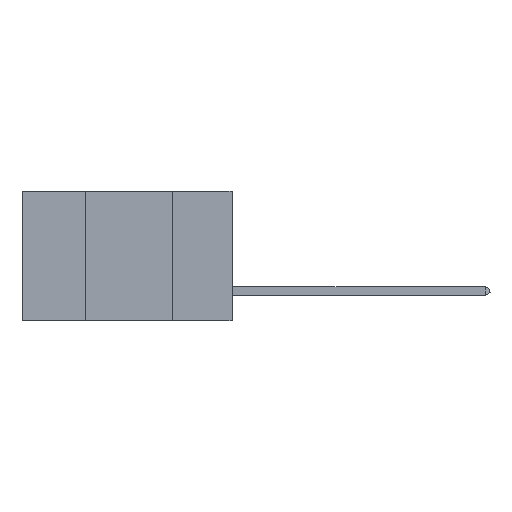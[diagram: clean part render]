
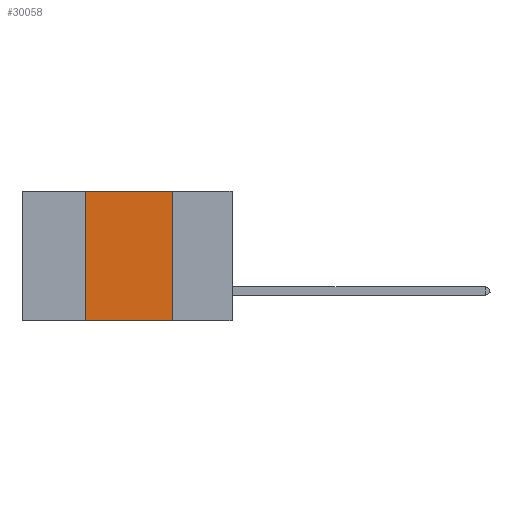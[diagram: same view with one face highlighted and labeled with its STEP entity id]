
A CAD part, left-side view. The second image highlights one B-rep face of the part: STEP entity #30058.
In plain terms, the highlighted planar face has unit normal (-1, 0, 0).
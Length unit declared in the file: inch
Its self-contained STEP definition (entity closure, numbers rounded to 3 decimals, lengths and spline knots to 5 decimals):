
#289 = VERTEX_POINT ( 'NONE', #24960 ) ;
#2509 = DIRECTION ( 'NONE',  ( 0., 0., 1. ) ) ;
#3548 = DIRECTION ( 'NONE',  ( 1., 0., 0. ) ) ;
#4126 = CARTESIAN_POINT ( 'NONE',  ( 0., 0.42, 0. ) ) ;
#5103 = ORIENTED_EDGE ( 'NONE', *, *, #31413, .F. ) ;
#5664 = LINE ( 'NONE', #14095, #44110 ) ;
#5711 = CARTESIAN_POINT ( 'NONE',  ( 0., 0.6, 0. ) ) ;
#10487 = VECTOR ( 'NONE', #16768, 39.37008 ) ;
#10623 = EDGE_LOOP ( 'NONE', ( #30626, #41800, #5103, #26706 ) ) ;
#14095 = CARTESIAN_POINT ( 'NONE',  ( 0., 0.42, 0. ) ) ;
#14500 = DIRECTION ( 'NONE',  ( 0., 0., -1. ) ) ;
#16768 = DIRECTION ( 'NONE',  ( 0., 0., -1. ) ) ;
#18489 = VERTEX_POINT ( 'NONE', #28493 ) ;
#20964 = EDGE_CURVE ( 'NONE', #289, #18489, #33792, .T. ) ;
#22131 = CARTESIAN_POINT ( 'NONE',  ( 0., 0.6, 0. ) ) ;
#24960 = CARTESIAN_POINT ( 'NONE',  ( 0., 0.17, 0. ) ) ;
#25874 = PLANE ( 'NONE',  #47348 ) ;
#26318 = CARTESIAN_POINT ( 'NONE',  ( 0., 0.6, -0.37 ) ) ;
#26706 = ORIENTED_EDGE ( 'NONE', *, *, #45067, .T. ) ;
#26965 = VECTOR ( 'NONE', #35706, 39.37008 ) ;
#28493 = CARTESIAN_POINT ( 'NONE',  ( 0., 0.17, -0.37 ) ) ;
#28886 = VERTEX_POINT ( 'NONE', #45642 ) ;
#29574 = DIRECTION ( 'NONE',  ( 0., -1., 0. ) ) ;
#30058 = ADVANCED_FACE ( 'NONE', ( #30864 ), #25874, .F. ) ;
#30626 = ORIENTED_EDGE ( 'NONE', *, *, #20964, .F. ) ;
#30864 = FACE_OUTER_BOUND ( 'NONE', #10623, .T. ) ;
#31413 = EDGE_CURVE ( 'NONE', #28886, #35418, #5664, .T. ) ;
#33792 = LINE ( 'NONE', #42944, #10487 ) ;
#35418 = VERTEX_POINT ( 'NONE', #4126 ) ;
#35706 = DIRECTION ( 'NONE',  ( 0., -1., 0. ) ) ;
#36193 = VECTOR ( 'NONE', #29574, 39.37008 ) ;
#39775 = LINE ( 'NONE', #5711, #26965 ) ;
#41800 = ORIENTED_EDGE ( 'NONE', *, *, #44244, .F. ) ;
#42944 = CARTESIAN_POINT ( 'NONE',  ( 0., 0.17, 0. ) ) ;
#44110 = VECTOR ( 'NONE', #2509, 39.37008 ) ;
#44244 = EDGE_CURVE ( 'NONE', #35418, #289, #39775, .T. ) ;
#45067 = EDGE_CURVE ( 'NONE', #28886, #18489, #47229, .T. ) ;
#45642 = CARTESIAN_POINT ( 'NONE',  ( 0., 0.42, -0.37 ) ) ;
#47229 = LINE ( 'NONE', #26318, #36193 ) ;
#47348 = AXIS2_PLACEMENT_3D ( 'NONE', #22131, #3548, #14500 ) ;
